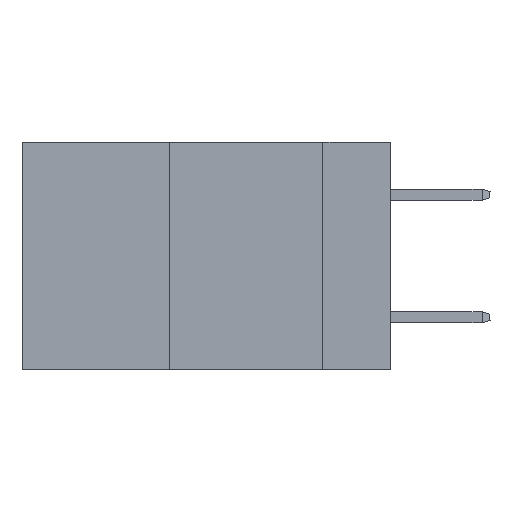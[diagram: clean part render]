
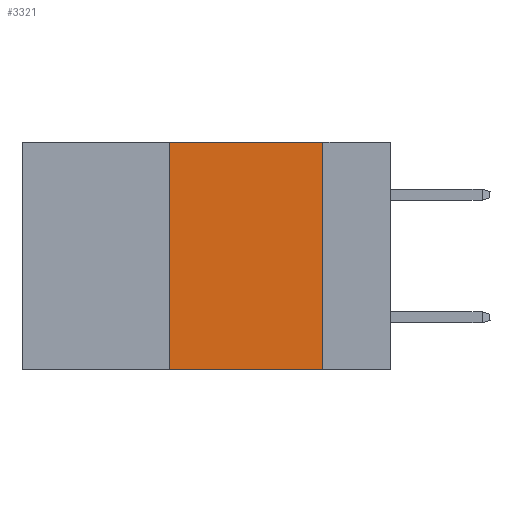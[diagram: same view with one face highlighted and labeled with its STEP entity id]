
A CAD part, left-side view. The second image highlights one B-rep face of the part: STEP entity #3321.
In plain terms, the highlighted planar face has unit normal (-1, 0, 0).
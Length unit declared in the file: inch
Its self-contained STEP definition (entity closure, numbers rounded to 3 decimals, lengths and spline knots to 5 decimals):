
#1824 = VECTOR ( 'NONE', #15473, 39.37008 ) ;
#2666 = VECTOR ( 'NONE', #2923, 39.37008 ) ;
#2923 = DIRECTION ( 'NONE',  ( 0., -1., 0. ) ) ;
#3321 = ADVANCED_FACE ( 'NONE', ( #28608 ), #33340, .F. ) ;
#3584 = CARTESIAN_POINT ( 'NONE',  ( 0., 0.6, 0. ) ) ;
#5327 = ORIENTED_EDGE ( 'NONE', *, *, #17813, .F. ) ;
#5494 = ORIENTED_EDGE ( 'NONE', *, *, #33662, .T. ) ;
#9511 = VECTOR ( 'NONE', #39679, 39.37008 ) ;
#10910 = DIRECTION ( 'NONE',  ( 0., 0., -1. ) ) ;
#11704 = VERTEX_POINT ( 'NONE', #26698 ) ;
#14084 = AXIS2_PLACEMENT_3D ( 'NONE', #15352, #31375, #24994 ) ;
#14569 = CARTESIAN_POINT ( 'NONE',  ( 0., 0.36, 0. ) ) ;
#14820 = VECTOR ( 'NONE', #10910, 39.37008 ) ;
#15352 = CARTESIAN_POINT ( 'NONE',  ( 0., 0.6, 0. ) ) ;
#15473 = DIRECTION ( 'NONE',  ( 0., -1., 0. ) ) ;
#16447 = VERTEX_POINT ( 'NONE', #14569 ) ;
#17813 = EDGE_CURVE ( 'NONE', #29672, #37443, #28622, .T. ) ;
#18618 = CARTESIAN_POINT ( 'NONE',  ( 0., 0.11, -0.37 ) ) ;
#21356 = LINE ( 'NONE', #33893, #9511 ) ;
#21819 = ORIENTED_EDGE ( 'NONE', *, *, #26837, .F. ) ;
#22615 = EDGE_LOOP ( 'NONE', ( #5327, #29247, #21819, #5494 ) ) ;
#24994 = DIRECTION ( 'NONE',  ( 0., 0., -1. ) ) ;
#26698 = CARTESIAN_POINT ( 'NONE',  ( 0., 0.36, -0.37 ) ) ;
#26837 = EDGE_CURVE ( 'NONE', #11704, #16447, #21356, .T. ) ;
#27799 = LINE ( 'NONE', #3584, #2666 ) ;
#28163 = CARTESIAN_POINT ( 'NONE',  ( 0., 0.6, -0.37 ) ) ;
#28608 = FACE_OUTER_BOUND ( 'NONE', #22615, .T. ) ;
#28622 = LINE ( 'NONE', #29819, #14820 ) ;
#29247 = ORIENTED_EDGE ( 'NONE', *, *, #36309, .F. ) ;
#29672 = VERTEX_POINT ( 'NONE', #33866 ) ;
#29819 = CARTESIAN_POINT ( 'NONE',  ( 0., 0.11, 0. ) ) ;
#31375 = DIRECTION ( 'NONE',  ( 1., 0., 0. ) ) ;
#33340 = PLANE ( 'NONE',  #14084 ) ;
#33662 = EDGE_CURVE ( 'NONE', #11704, #37443, #38326, .T. ) ;
#33866 = CARTESIAN_POINT ( 'NONE',  ( 0., 0.11, 0. ) ) ;
#33893 = CARTESIAN_POINT ( 'NONE',  ( 0., 0.36, 0. ) ) ;
#36309 = EDGE_CURVE ( 'NONE', #16447, #29672, #27799, .T. ) ;
#37443 = VERTEX_POINT ( 'NONE', #18618 ) ;
#38326 = LINE ( 'NONE', #28163, #1824 ) ;
#39679 = DIRECTION ( 'NONE',  ( 0., 0., 1. ) ) ;
